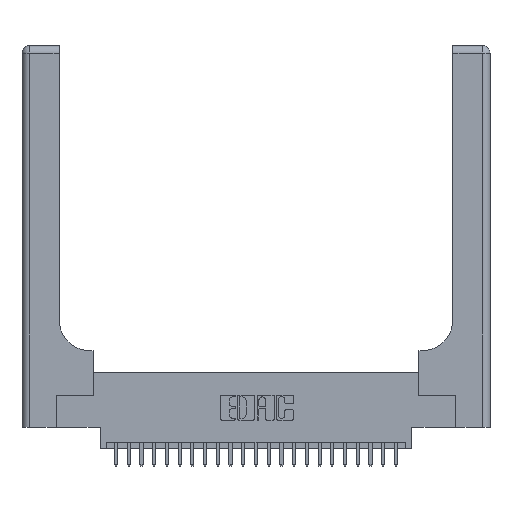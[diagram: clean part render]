
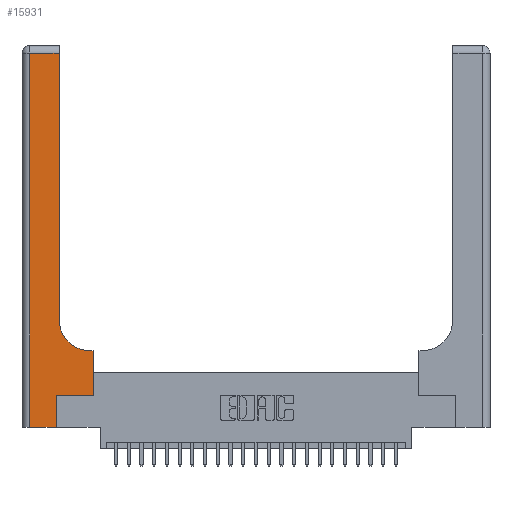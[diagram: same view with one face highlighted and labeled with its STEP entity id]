
A CAD part, top view. The second image highlights one B-rep face of the part: STEP entity #15931.
In plain terms, the highlighted planar face has unit normal (0, 0, 1).
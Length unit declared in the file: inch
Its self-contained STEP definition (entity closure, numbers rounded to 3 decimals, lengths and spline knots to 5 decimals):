
#1104 = CARTESIAN_POINT ( 'NONE',  ( 0.5585, 0.25, 0.37 ) ) ;
#1175 = VECTOR ( 'NONE', #23008, 39.37008 ) ;
#1435 = CARTESIAN_POINT ( 'NONE',  ( 0.269, 0., 0.37 ) ) ;
#2817 = CARTESIAN_POINT ( 'NONE',  ( 0.06, 0., 0.37 ) ) ;
#2977 = AXIS2_PLACEMENT_3D ( 'NONE', #8861, #17234, #25071 ) ;
#3452 = EDGE_CURVE ( 'NONE', #24897, #12071, #11264, .T. ) ;
#3760 = VERTEX_POINT ( 'NONE', #12980 ) ;
#4493 = EDGE_CURVE ( 'NONE', #8207, #7301, #22797, .T. ) ;
#4621 = VECTOR ( 'NONE', #17182, 39.37008 ) ;
#5285 = CARTESIAN_POINT ( 'NONE',  ( 0.5585, 0.6, 0.37 ) ) ;
#5883 = DIRECTION ( 'NONE',  ( 0., 0., -1. ) ) ;
#7021 = FACE_OUTER_BOUND ( 'NONE', #12682, .T. ) ;
#7216 = ORIENTED_EDGE ( 'NONE', *, *, #16810, .T. ) ;
#7301 = VERTEX_POINT ( 'NONE', #2817 ) ;
#7900 = VECTOR ( 'NONE', #13356, 39.37008 ) ;
#7974 = VECTOR ( 'NONE', #24915, 39.37008 ) ;
#8184 = ORIENTED_EDGE ( 'NONE', *, *, #13607, .T. ) ;
#8207 = VERTEX_POINT ( 'NONE', #17262 ) ;
#8861 = CARTESIAN_POINT ( 'NONE',  ( 0.5415, 0.85, 0.37 ) ) ;
#8867 = EDGE_CURVE ( 'NONE', #3760, #24897, #14554, .T. ) ;
#9602 = ORIENTED_EDGE ( 'NONE', *, *, #12050, .T. ) ;
#10213 = ORIENTED_EDGE ( 'NONE', *, *, #20186, .T. ) ;
#11264 = LINE ( 'NONE', #1104, #4621 ) ;
#11538 = DIRECTION ( 'NONE',  ( -1., 0., 0. ) ) ;
#12050 = EDGE_CURVE ( 'NONE', #24442, #8207, #13146, .T. ) ;
#12071 = VERTEX_POINT ( 'NONE', #5285 ) ;
#12171 = ORIENTED_EDGE ( 'NONE', *, *, #12637, .T. ) ;
#12637 = EDGE_CURVE ( 'NONE', #12071, #23525, #16255, .T. ) ;
#12682 = EDGE_LOOP ( 'NONE', ( #10213, #9602, #23267, #7216, #20555, #15562, #23886, #12171, #8184 ) ) ;
#12718 = CARTESIAN_POINT ( 'NONE',  ( 0.2915, 0.6, 0.37 ) ) ;
#12936 = AXIS2_PLACEMENT_3D ( 'NONE', #24312, #5883, #17137 ) ;
#12980 = CARTESIAN_POINT ( 'NONE',  ( 0.269, 0.25, 0.37 ) ) ;
#13146 = LINE ( 'NONE', #21382, #23187 ) ;
#13356 = DIRECTION ( 'NONE',  ( 0., 1., 0. ) ) ;
#13607 = EDGE_CURVE ( 'NONE', #23525, #19497, #20958, .T. ) ;
#14515 = VECTOR ( 'NONE', #22662, 39.37008 ) ;
#14554 = LINE ( 'NONE', #20745, #7974 ) ;
#15170 = LINE ( 'NONE', #24494, #14515 ) ;
#15562 = ORIENTED_EDGE ( 'NONE', *, *, #8867, .T. ) ;
#15931 = ADVANCED_FACE ( 'NONE', ( #7021 ), #19885, .F. ) ;
#16222 = CARTESIAN_POINT ( 'NONE',  ( 0.06, 3., 0.37 ) ) ;
#16255 = LINE ( 'NONE', #12718, #1175 ) ;
#16810 = EDGE_CURVE ( 'NONE', #7301, #18402, #15170, .T. ) ;
#16864 = VECTOR ( 'NONE', #22184, 39.37008 ) ;
#17137 = DIRECTION ( 'NONE',  ( -1., 0., 0. ) ) ;
#17182 = DIRECTION ( 'NONE',  ( 0., 1., 0. ) ) ;
#17234 = DIRECTION ( 'NONE',  ( 0., 0., -1. ) ) ;
#17262 = CARTESIAN_POINT ( 'NONE',  ( 0.06, 2.94, 0.37 ) ) ;
#17462 = VECTOR ( 'NONE', #24516, 39.37008 ) ;
#18402 = VERTEX_POINT ( 'NONE', #25680 ) ;
#19497 = VERTEX_POINT ( 'NONE', #20125 ) ;
#19885 = PLANE ( 'NONE',  #12936 ) ;
#20125 = CARTESIAN_POINT ( 'NONE',  ( 0.2915, 0.85, 0.37 ) ) ;
#20186 = EDGE_CURVE ( 'NONE', #19497, #24442, #22751, .T. ) ;
#20555 = ORIENTED_EDGE ( 'NONE', *, *, #22431, .T. ) ;
#20745 = CARTESIAN_POINT ( 'NONE',  ( 0.269, 0.25, 0.37 ) ) ;
#20958 = CIRCLE ( 'NONE', #2977, 0.25 ) ;
#21313 = CARTESIAN_POINT ( 'NONE',  ( 0.5415, 0.6, 0.37 ) ) ;
#21382 = CARTESIAN_POINT ( 'NONE',  ( 0., 2.94, 0.37 ) ) ;
#21963 = CARTESIAN_POINT ( 'NONE',  ( 0.2915, 2.94, 0.37 ) ) ;
#22184 = DIRECTION ( 'NONE',  ( 0., -1., 0. ) ) ;
#22241 = CARTESIAN_POINT ( 'NONE',  ( 0.5585, 0.25, 0.37 ) ) ;
#22431 = EDGE_CURVE ( 'NONE', #18402, #3760, #25453, .T. ) ;
#22662 = DIRECTION ( 'NONE',  ( 1., 0., 0. ) ) ;
#22751 = LINE ( 'NONE', #22771, #17462 ) ;
#22771 = CARTESIAN_POINT ( 'NONE',  ( 0.2915, 3., 0.37 ) ) ;
#22797 = LINE ( 'NONE', #16222, #16864 ) ;
#23008 = DIRECTION ( 'NONE',  ( -1., 0., 0. ) ) ;
#23187 = VECTOR ( 'NONE', #11538, 39.37008 ) ;
#23267 = ORIENTED_EDGE ( 'NONE', *, *, #4493, .T. ) ;
#23525 = VERTEX_POINT ( 'NONE', #21313 ) ;
#23886 = ORIENTED_EDGE ( 'NONE', *, *, #3452, .T. ) ;
#24312 = CARTESIAN_POINT ( 'NONE',  ( 0., 3., 0.37 ) ) ;
#24442 = VERTEX_POINT ( 'NONE', #21963 ) ;
#24494 = CARTESIAN_POINT ( 'NONE',  ( 0., 0., 0.37 ) ) ;
#24516 = DIRECTION ( 'NONE',  ( 0., 1., 0. ) ) ;
#24897 = VERTEX_POINT ( 'NONE', #22241 ) ;
#24915 = DIRECTION ( 'NONE',  ( 1., 0., 0. ) ) ;
#25071 = DIRECTION ( 'NONE',  ( 1., 0., 0. ) ) ;
#25453 = LINE ( 'NONE', #1435, #7900 ) ;
#25680 = CARTESIAN_POINT ( 'NONE',  ( 0.269, 0., 0.37 ) ) ;
